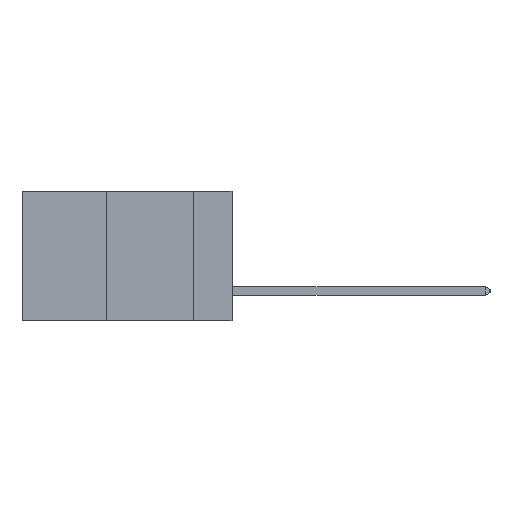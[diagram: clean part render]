
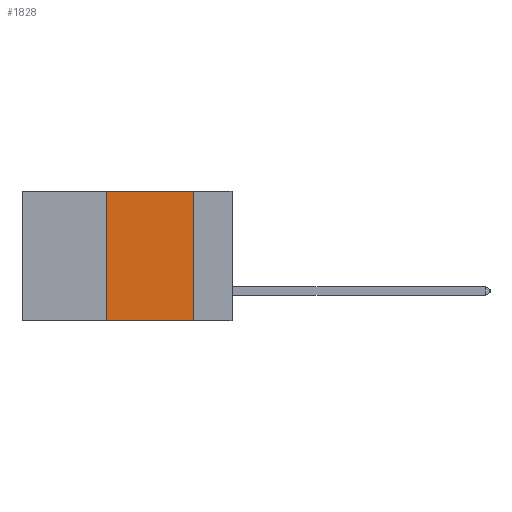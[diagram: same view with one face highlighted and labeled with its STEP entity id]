
A CAD part, left-side view. The second image highlights one B-rep face of the part: STEP entity #1828.
In plain terms, the highlighted planar face has unit normal (-1, 0, 0).
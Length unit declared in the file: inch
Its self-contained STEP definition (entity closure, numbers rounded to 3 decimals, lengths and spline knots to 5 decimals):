
#39 = EDGE_LOOP ( 'NONE', ( #17820, #23386, #9121, #19549 ) ) ;
#74 = PLANE ( 'NONE',  #6103 ) ;
#341 = LINE ( 'NONE', #12508, #19687 ) ;
#958 = VERTEX_POINT ( 'NONE', #14091 ) ;
#1442 = CARTESIAN_POINT ( 'NONE',  ( 0., 0.11, 0. ) ) ;
#1594 = CARTESIAN_POINT ( 'NONE',  ( 0., 0.6, -0.37 ) ) ;
#1828 = ADVANCED_FACE ( 'NONE', ( #24294 ), #74, .F. ) ;
#4047 = CARTESIAN_POINT ( 'NONE',  ( 0., 0.6, 0. ) ) ;
#4767 = LINE ( 'NONE', #10973, #9188 ) ;
#5858 = CARTESIAN_POINT ( 'NONE',  ( 0., 0.6, 0. ) ) ;
#6103 = AXIS2_PLACEMENT_3D ( 'NONE', #5858, #18845, #7750 ) ;
#6850 = DIRECTION ( 'NONE',  ( 0., 0., 1. ) ) ;
#7750 = DIRECTION ( 'NONE',  ( 0., 0., -1. ) ) ;
#7998 = LINE ( 'NONE', #1594, #23778 ) ;
#8154 = VERTEX_POINT ( 'NONE', #9179 ) ;
#8235 = LINE ( 'NONE', #4047, #23090 ) ;
#8518 = VERTEX_POINT ( 'NONE', #12360 ) ;
#9121 = ORIENTED_EDGE ( 'NONE', *, *, #11860, .F. ) ;
#9179 = CARTESIAN_POINT ( 'NONE',  ( 0., 0.36, -0.37 ) ) ;
#9188 = VECTOR ( 'NONE', #23976, 39.37008 ) ;
#9204 = DIRECTION ( 'NONE',  ( 0., -1., 0. ) ) ;
#9353 = EDGE_CURVE ( 'NONE', #8154, #8518, #7998, .T. ) ;
#10973 = CARTESIAN_POINT ( 'NONE',  ( 0., 0.11, 0. ) ) ;
#11860 = EDGE_CURVE ( 'NONE', #8154, #958, #341, .T. ) ;
#12360 = CARTESIAN_POINT ( 'NONE',  ( 0., 0.11, -0.37 ) ) ;
#12508 = CARTESIAN_POINT ( 'NONE',  ( 0., 0.36, 0. ) ) ;
#13136 = EDGE_CURVE ( 'NONE', #20121, #8518, #4767, .T. ) ;
#14091 = CARTESIAN_POINT ( 'NONE',  ( 0., 0.36, 0. ) ) ;
#17820 = ORIENTED_EDGE ( 'NONE', *, *, #13136, .F. ) ;
#18845 = DIRECTION ( 'NONE',  ( 1., 0., 0. ) ) ;
#18937 = DIRECTION ( 'NONE',  ( 0., -1., 0. ) ) ;
#19549 = ORIENTED_EDGE ( 'NONE', *, *, #9353, .T. ) ;
#19687 = VECTOR ( 'NONE', #6850, 39.37008 ) ;
#20121 = VERTEX_POINT ( 'NONE', #1442 ) ;
#23090 = VECTOR ( 'NONE', #18937, 39.37008 ) ;
#23386 = ORIENTED_EDGE ( 'NONE', *, *, #23397, .F. ) ;
#23397 = EDGE_CURVE ( 'NONE', #958, #20121, #8235, .T. ) ;
#23778 = VECTOR ( 'NONE', #9204, 39.37008 ) ;
#23976 = DIRECTION ( 'NONE',  ( 0., 0., -1. ) ) ;
#24294 = FACE_OUTER_BOUND ( 'NONE', #39, .T. ) ;
